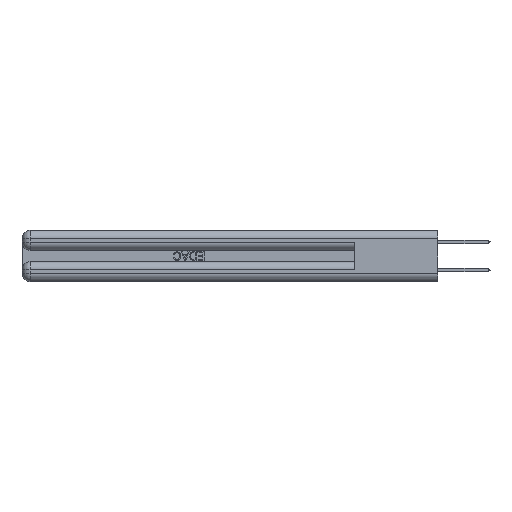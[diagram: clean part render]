
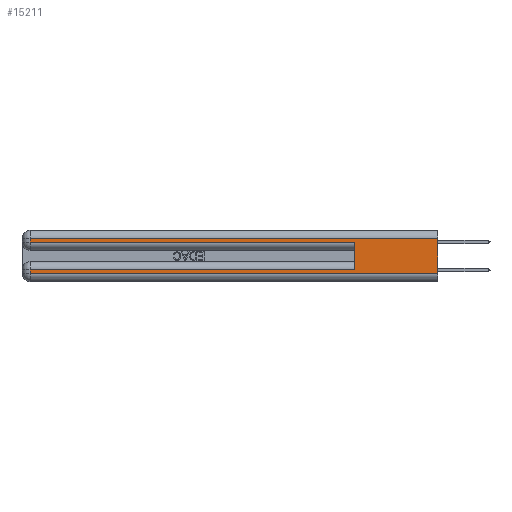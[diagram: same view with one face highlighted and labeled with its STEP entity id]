
A CAD part, left-side view. The second image highlights one B-rep face of the part: STEP entity #15211.
In plain terms, the highlighted planar face has unit normal (-1, 0, 0).
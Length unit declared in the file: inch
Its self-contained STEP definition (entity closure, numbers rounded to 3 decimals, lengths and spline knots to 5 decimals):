
#158 = EDGE_CURVE ( 'NONE', #34545, #28274, #26381, .T. ) ;
#561 = VERTEX_POINT ( 'NONE', #4377 ) ;
#2308 = LINE ( 'NONE', #14914, #40052 ) ;
#2330 = VECTOR ( 'NONE', #15763, 39.37008 ) ;
#3753 = VECTOR ( 'NONE', #15059, 39.37008 ) ;
#4377 = CARTESIAN_POINT ( 'NONE',  ( 0., 2.94, 0.285 ) ) ;
#5500 = PLANE ( 'NONE',  #39973 ) ;
#6315 = ORIENTED_EDGE ( 'NONE', *, *, #11382, .T. ) ;
#6377 = CARTESIAN_POINT ( 'NONE',  ( 0., 0., 0.085 ) ) ;
#6883 = LINE ( 'NONE', #6377, #14977 ) ;
#7183 = VERTEX_POINT ( 'NONE', #33492 ) ;
#7753 = VERTEX_POINT ( 'NONE', #33452 ) ;
#8591 = CARTESIAN_POINT ( 'NONE',  ( 0., 2.94, 0.37 ) ) ;
#8714 = LINE ( 'NONE', #22551, #35098 ) ;
#8979 = DIRECTION ( 'NONE',  ( 0., 0., -1. ) ) ;
#9026 = ORIENTED_EDGE ( 'NONE', *, *, #158, .F. ) ;
#10473 = LINE ( 'NONE', #8591, #18612 ) ;
#10649 = FACE_OUTER_BOUND ( 'NONE', #27504, .T. ) ;
#11382 = EDGE_CURVE ( 'NONE', #20211, #561, #10473, .T. ) ;
#11612 = CARTESIAN_POINT ( 'NONE',  ( 0., 0., 0.31 ) ) ;
#12775 = ORIENTED_EDGE ( 'NONE', *, *, #24063, .T. ) ;
#12893 = CARTESIAN_POINT ( 'NONE',  ( 0., 0.6, 0.145 ) ) ;
#12989 = LINE ( 'NONE', #11612, #3753 ) ;
#13311 = EDGE_CURVE ( 'NONE', #42446, #20211, #12989, .T. ) ;
#14914 = CARTESIAN_POINT ( 'NONE',  ( 0., 0., 0.285 ) ) ;
#14977 = VECTOR ( 'NONE', #27076, 39.37008 ) ;
#15059 = DIRECTION ( 'NONE',  ( 0., 1., 0. ) ) ;
#15211 = ADVANCED_FACE ( 'NONE', ( #10649 ), #5500, .F. ) ;
#15763 = DIRECTION ( 'NONE',  ( 0., -1., 0. ) ) ;
#17413 = CARTESIAN_POINT ( 'NONE',  ( 0., 2.94, 0.37 ) ) ;
#18612 = VECTOR ( 'NONE', #36099, 39.37008 ) ;
#18768 = ORIENTED_EDGE ( 'NONE', *, *, #26251, .T. ) ;
#19260 = CARTESIAN_POINT ( 'NONE',  ( 0., 0.6, 0.285 ) ) ;
#20211 = VERTEX_POINT ( 'NONE', #44292 ) ;
#21420 = EDGE_CURVE ( 'NONE', #7183, #7753, #39891, .T. ) ;
#21743 = EDGE_CURVE ( 'NONE', #42446, #32667, #8714, .T. ) ;
#21976 = CARTESIAN_POINT ( 'NONE',  ( 0., 0., 0.31 ) ) ;
#22551 = CARTESIAN_POINT ( 'NONE',  ( 0., 0., 0.37 ) ) ;
#22783 = CARTESIAN_POINT ( 'NONE',  ( 0., 0., 0.37 ) ) ;
#24063 = EDGE_CURVE ( 'NONE', #34545, #7183, #6883, .T. ) ;
#25312 = VECTOR ( 'NONE', #30075, 39.37008 ) ;
#26251 = EDGE_CURVE ( 'NONE', #7753, #32667, #28888, .T. ) ;
#26381 = LINE ( 'NONE', #12893, #25312 ) ;
#27076 = DIRECTION ( 'NONE',  ( 0., 1., 0. ) ) ;
#27504 = EDGE_LOOP ( 'NONE', ( #34411, #38614, #6315, #28418, #9026, #12775, #43331, #18768 ) ) ;
#28274 = VERTEX_POINT ( 'NONE', #19260 ) ;
#28418 = ORIENTED_EDGE ( 'NONE', *, *, #44406, .T. ) ;
#28888 = LINE ( 'NONE', #36333, #2330 ) ;
#29567 = DIRECTION ( 'NONE',  ( 0., 0., -1. ) ) ;
#30075 = DIRECTION ( 'NONE',  ( 0., 0., 1. ) ) ;
#30861 = VECTOR ( 'NONE', #41349, 39.37008 ) ;
#32667 = VERTEX_POINT ( 'NONE', #40590 ) ;
#33452 = CARTESIAN_POINT ( 'NONE',  ( 0., 2.94, 0.06 ) ) ;
#33492 = CARTESIAN_POINT ( 'NONE',  ( 0., 2.94, 0.085 ) ) ;
#34411 = ORIENTED_EDGE ( 'NONE', *, *, #21743, .F. ) ;
#34545 = VERTEX_POINT ( 'NONE', #36452 ) ;
#35098 = VECTOR ( 'NONE', #29567, 39.37008 ) ;
#36099 = DIRECTION ( 'NONE',  ( 0., 0., -1. ) ) ;
#36333 = CARTESIAN_POINT ( 'NONE',  ( 0., 0., 0.06 ) ) ;
#36452 = CARTESIAN_POINT ( 'NONE',  ( 0., 0.6, 0.085 ) ) ;
#38614 = ORIENTED_EDGE ( 'NONE', *, *, #13311, .T. ) ;
#38931 = DIRECTION ( 'NONE',  ( 0., -1., 0. ) ) ;
#39891 = LINE ( 'NONE', #17413, #30861 ) ;
#39973 = AXIS2_PLACEMENT_3D ( 'NONE', #22783, #43187, #8979 ) ;
#40052 = VECTOR ( 'NONE', #38931, 39.37008 ) ;
#40590 = CARTESIAN_POINT ( 'NONE',  ( 0., 0., 0.06 ) ) ;
#41349 = DIRECTION ( 'NONE',  ( 0., 0., -1. ) ) ;
#42446 = VERTEX_POINT ( 'NONE', #21976 ) ;
#43187 = DIRECTION ( 'NONE',  ( 1., 0., 0. ) ) ;
#43331 = ORIENTED_EDGE ( 'NONE', *, *, #21420, .T. ) ;
#44292 = CARTESIAN_POINT ( 'NONE',  ( 0., 2.94, 0.31 ) ) ;
#44406 = EDGE_CURVE ( 'NONE', #561, #28274, #2308, .T. ) ;
